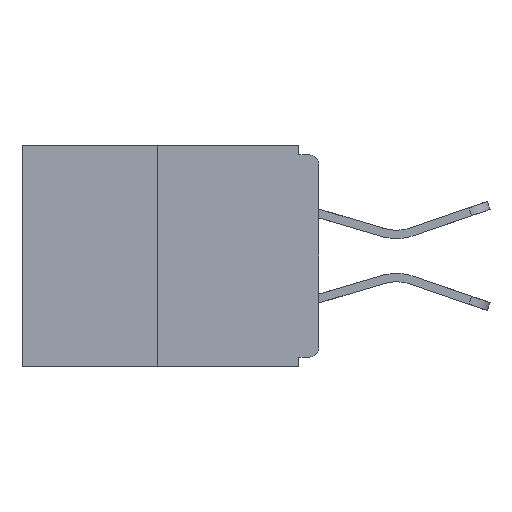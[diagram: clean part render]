
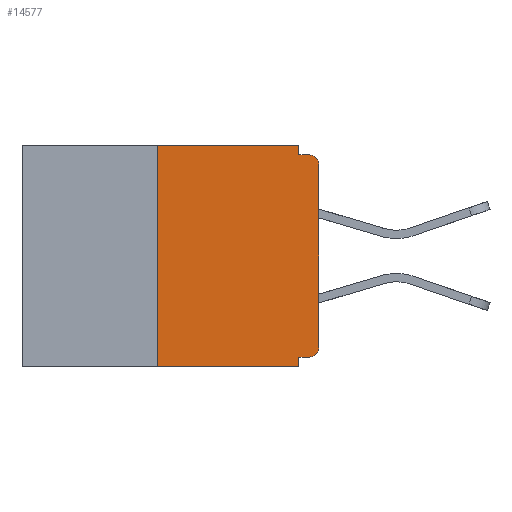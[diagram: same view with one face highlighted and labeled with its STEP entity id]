
A CAD part, left-side view. The second image highlights one B-rep face of the part: STEP entity #14577.
In plain terms, the highlighted planar face has unit normal (-1, 0, 0).
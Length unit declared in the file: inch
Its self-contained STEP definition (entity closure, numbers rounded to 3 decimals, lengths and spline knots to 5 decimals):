
#647 = ORIENTED_EDGE ( 'NONE', *, *, #13481, .T. ) ;
#963 = DIRECTION ( 'NONE',  ( 0., 0., -1. ) ) ;
#1195 = AXIS2_PLACEMENT_3D ( 'NONE', #7940, #22076, #7829 ) ;
#1864 = DIRECTION ( 'NONE',  ( 0., 1., 0. ) ) ;
#2005 = CIRCLE ( 'NONE', #1195, 0.015 ) ;
#2077 = CARTESIAN_POINT ( 'NONE',  ( 0., 0., -0.03 ) ) ;
#2181 = VECTOR ( 'NONE', #3386, 39.37008 ) ;
#2259 = CARTESIAN_POINT ( 'NONE',  ( 0., 0.25, 0. ) ) ;
#2448 = EDGE_CURVE ( 'NONE', #29203, #26162, #8888, .T. ) ;
#2453 = AXIS2_PLACEMENT_3D ( 'NONE', #9266, #6996, #18691 ) ;
#3386 = DIRECTION ( 'NONE',  ( 0., -1., 0. ) ) ;
#3688 = EDGE_LOOP ( 'NONE', ( #4131, #7533, #647, #9476, #15260, #24077, #25593, #11080, #6270, #26115 ) ) ;
#4131 = ORIENTED_EDGE ( 'NONE', *, *, #15996, .F. ) ;
#4634 = CARTESIAN_POINT ( 'NONE',  ( 0., 0.46, 0. ) ) ;
#4861 = LINE ( 'NONE', #2259, #15408 ) ;
#6160 = CARTESIAN_POINT ( 'NONE',  ( 0., 0.015, -0.015 ) ) ;
#6270 = ORIENTED_EDGE ( 'NONE', *, *, #18659, .F. ) ;
#6640 = DIRECTION ( 'NONE',  ( 1., 0., 0. ) ) ;
#6996 = DIRECTION ( 'NONE',  ( -1., 0., 0. ) ) ;
#7037 = LINE ( 'NONE', #9170, #24828 ) ;
#7533 = ORIENTED_EDGE ( 'NONE', *, *, #21866, .F. ) ;
#7591 = LINE ( 'NONE', #4634, #2181 ) ;
#7823 = VERTEX_POINT ( 'NONE', #24871 ) ;
#7829 = DIRECTION ( 'NONE',  ( 0., 0., -1. ) ) ;
#7940 = CARTESIAN_POINT ( 'NONE',  ( 0., 0.015, -0.313 ) ) ;
#8888 = LINE ( 'NONE', #19536, #28422 ) ;
#9117 = EDGE_CURVE ( 'NONE', #12628, #27573, #11683, .T. ) ;
#9170 = CARTESIAN_POINT ( 'NONE',  ( 0., 0., 0. ) ) ;
#9266 = CARTESIAN_POINT ( 'NONE',  ( 0., 0.015, -0.03 ) ) ;
#9383 = LINE ( 'NONE', #23571, #19185 ) ;
#9476 = ORIENTED_EDGE ( 'NONE', *, *, #2448, .F. ) ;
#9564 = VERTEX_POINT ( 'NONE', #15414 ) ;
#10013 = EDGE_CURVE ( 'NONE', #9564, #29203, #27884, .T. ) ;
#10693 = CARTESIAN_POINT ( 'NONE',  ( 0., 0.031, -0.328 ) ) ;
#11035 = CARTESIAN_POINT ( 'NONE',  ( 0., 0.25, 0. ) ) ;
#11080 = ORIENTED_EDGE ( 'NONE', *, *, #9117, .T. ) ;
#11143 = PLANE ( 'NONE',  #11303 ) ;
#11303 = AXIS2_PLACEMENT_3D ( 'NONE', #22713, #6640, #15605 ) ;
#11683 = CIRCLE ( 'NONE', #2453, 0.015 ) ;
#11854 = DIRECTION ( 'NONE',  ( 0., 0., -1. ) ) ;
#12628 = VERTEX_POINT ( 'NONE', #2077 ) ;
#13481 = EDGE_CURVE ( 'NONE', #15137, #26162, #15694, .T. ) ;
#13578 = CARTESIAN_POINT ( 'NONE',  ( 0., 0.031, -0.015 ) ) ;
#13639 = CARTESIAN_POINT ( 'NONE',  ( 0., 0., -0.328 ) ) ;
#13806 = CARTESIAN_POINT ( 'NONE',  ( 0., 0.25, -0.343 ) ) ;
#14146 = LINE ( 'NONE', #25793, #26047 ) ;
#14577 = ADVANCED_FACE ( 'NONE', ( #27933 ), #11143, .F. ) ;
#14588 = VERTEX_POINT ( 'NONE', #11035 ) ;
#15137 = VERTEX_POINT ( 'NONE', #13806 ) ;
#15260 = ORIENTED_EDGE ( 'NONE', *, *, #10013, .F. ) ;
#15408 = VECTOR ( 'NONE', #20514, 39.37008 ) ;
#15414 = CARTESIAN_POINT ( 'NONE',  ( 0., 0.015, -0.328 ) ) ;
#15605 = DIRECTION ( 'NONE',  ( 0., 0., -1. ) ) ;
#15694 = LINE ( 'NONE', #19998, #23337 ) ;
#15996 = EDGE_CURVE ( 'NONE', #14588, #7823, #7591, .T. ) ;
#16148 = VERTEX_POINT ( 'NONE', #13578 ) ;
#16664 = DIRECTION ( 'NONE',  ( 0., -1., 0. ) ) ;
#18659 = EDGE_CURVE ( 'NONE', #16148, #27573, #9383, .T. ) ;
#18691 = DIRECTION ( 'NONE',  ( 0., 0., -1. ) ) ;
#19185 = VECTOR ( 'NONE', #16664, 39.37008 ) ;
#19536 = CARTESIAN_POINT ( 'NONE',  ( 0., 0.031, -0.343 ) ) ;
#19602 = DIRECTION ( 'NONE',  ( 0., -1., 0. ) ) ;
#19952 = VECTOR ( 'NONE', #1864, 39.37008 ) ;
#19998 = CARTESIAN_POINT ( 'NONE',  ( 0., 0.46, -0.343 ) ) ;
#20514 = DIRECTION ( 'NONE',  ( 0., 0., 1. ) ) ;
#21757 = CARTESIAN_POINT ( 'NONE',  ( 0., 0., -0.313 ) ) ;
#21787 = EDGE_CURVE ( 'NONE', #25206, #12628, #7037, .T. ) ;
#21866 = EDGE_CURVE ( 'NONE', #15137, #14588, #4861, .T. ) ;
#22076 = DIRECTION ( 'NONE',  ( -1., 0., 0. ) ) ;
#22173 = CARTESIAN_POINT ( 'NONE',  ( 0., 0.031, -0.343 ) ) ;
#22713 = CARTESIAN_POINT ( 'NONE',  ( 0., 0.46, 0. ) ) ;
#23281 = DIRECTION ( 'NONE',  ( 0., 0., 1. ) ) ;
#23337 = VECTOR ( 'NONE', #19602, 39.37008 ) ;
#23571 = CARTESIAN_POINT ( 'NONE',  ( 0., 0., -0.015 ) ) ;
#24077 = ORIENTED_EDGE ( 'NONE', *, *, #25189, .T. ) ;
#24828 = VECTOR ( 'NONE', #23281, 39.37008 ) ;
#24871 = CARTESIAN_POINT ( 'NONE',  ( 0., 0.031, 0. ) ) ;
#25189 = EDGE_CURVE ( 'NONE', #9564, #25206, #2005, .T. ) ;
#25206 = VERTEX_POINT ( 'NONE', #21757 ) ;
#25593 = ORIENTED_EDGE ( 'NONE', *, *, #21787, .T. ) ;
#25793 = CARTESIAN_POINT ( 'NONE',  ( 0., 0.031, 0. ) ) ;
#26047 = VECTOR ( 'NONE', #11854, 39.37008 ) ;
#26115 = ORIENTED_EDGE ( 'NONE', *, *, #29003, .F. ) ;
#26162 = VERTEX_POINT ( 'NONE', #22173 ) ;
#27573 = VERTEX_POINT ( 'NONE', #6160 ) ;
#27884 = LINE ( 'NONE', #13639, #19952 ) ;
#27933 = FACE_OUTER_BOUND ( 'NONE', #3688, .T. ) ;
#28422 = VECTOR ( 'NONE', #963, 39.37008 ) ;
#29003 = EDGE_CURVE ( 'NONE', #7823, #16148, #14146, .T. ) ;
#29203 = VERTEX_POINT ( 'NONE', #10693 ) ;
